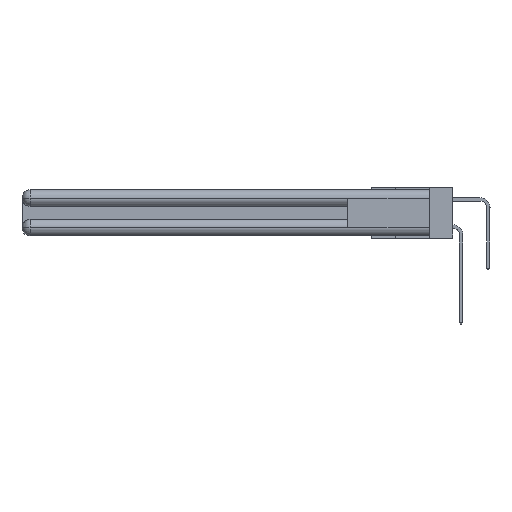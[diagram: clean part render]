
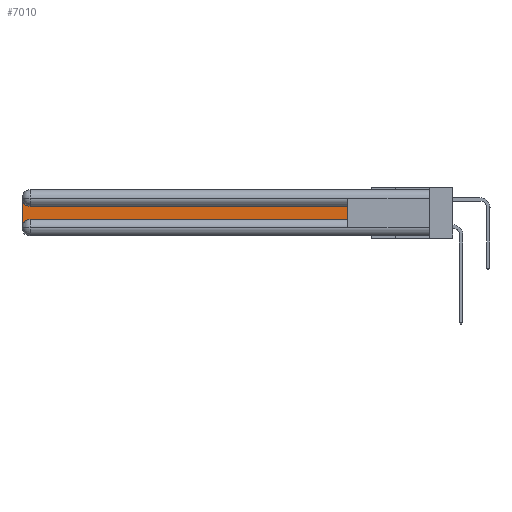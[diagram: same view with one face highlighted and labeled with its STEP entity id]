
A CAD part, left-side view. The second image highlights one B-rep face of the part: STEP entity #7010.
In plain terms, the highlighted planar face has unit normal (-1, 0, 0).
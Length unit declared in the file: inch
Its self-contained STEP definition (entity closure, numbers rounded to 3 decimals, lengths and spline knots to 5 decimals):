
#18 = DIRECTION ( 'NONE',  ( 1., 0., 0. ) ) ;
#355 = CARTESIAN_POINT ( 'NONE',  ( 0.075, 2.94, -0.2775 ) ) ;
#578 = CARTESIAN_POINT ( 'NONE',  ( 0.075, 2.94, -0.2175 ) ) ;
#766 = ORIENTED_EDGE ( 'NONE', *, *, #27899, .T. ) ;
#861 = EDGE_CURVE ( 'NONE', #5225, #5058, #1447, .T. ) ;
#911 = EDGE_CURVE ( 'NONE', #29922, #8010, #19215, .T. ) ;
#1120 = EDGE_CURVE ( 'NONE', #6606, #12666, #27124, .T. ) ;
#1179 = DIRECTION ( 'NONE',  ( 0., 0., 1. ) ) ;
#1447 = CIRCLE ( 'NONE', #16295, 0.06 ) ;
#1865 = CARTESIAN_POINT ( 'NONE',  ( 0.075, 3., -0.2175 ) ) ;
#2793 = DIRECTION ( 'NONE',  ( 1., 0., 0. ) ) ;
#4645 = ORIENTED_EDGE ( 'NONE', *, *, #19676, .T. ) ;
#4651 = FACE_OUTER_BOUND ( 'NONE', #5814, .T. ) ;
#5058 = VERTEX_POINT ( 'NONE', #7062 ) ;
#5225 = VERTEX_POINT ( 'NONE', #29302 ) ;
#5548 = DIRECTION ( 'NONE',  ( 0., 1., 0. ) ) ;
#5814 = EDGE_LOOP ( 'NONE', ( #4645, #27393, #766, #28518, #8249, #23352 ) ) ;
#6006 = CARTESIAN_POINT ( 'NONE',  ( 0.075, 0.6, -0.2175 ) ) ;
#6606 = VERTEX_POINT ( 'NONE', #13624 ) ;
#7010 = ADVANCED_FACE ( 'NONE', ( #4651 ), #20815, .F. ) ;
#7062 = CARTESIAN_POINT ( 'NONE',  ( 0.075, 3., -0.0625 ) ) ;
#8010 = VERTEX_POINT ( 'NONE', #578 ) ;
#8151 = AXIS2_PLACEMENT_3D ( 'NONE', #23577, #18272, #28086 ) ;
#8249 = ORIENTED_EDGE ( 'NONE', *, *, #24310, .T. ) ;
#9406 = CARTESIAN_POINT ( 'NONE',  ( 0.075, 3., -0.2775 ) ) ;
#11035 = VECTOR ( 'NONE', #5548, 39.37008 ) ;
#12666 = VERTEX_POINT ( 'NONE', #16071 ) ;
#13624 = CARTESIAN_POINT ( 'NONE',  ( 0.075, 0.6, -0.2175 ) ) ;
#16071 = CARTESIAN_POINT ( 'NONE',  ( 0.075, 0.6, -0.1225 ) ) ;
#16295 = AXIS2_PLACEMENT_3D ( 'NONE', #29096, #18, #22030 ) ;
#18272 = DIRECTION ( 'NONE',  ( 1., 0., 0. ) ) ;
#19215 = CIRCLE ( 'NONE', #22332, 0.06 ) ;
#19676 = EDGE_CURVE ( 'NONE', #12666, #5225, #26894, .T. ) ;
#20035 = CARTESIAN_POINT ( 'NONE',  ( 0.075, 0.6, -0.1225 ) ) ;
#20189 = LINE ( 'NONE', #24425, #22486 ) ;
#20815 = PLANE ( 'NONE',  #8151 ) ;
#21258 = LINE ( 'NONE', #1865, #27285 ) ;
#21796 = DIRECTION ( 'NONE',  ( 0., -1., 0. ) ) ;
#22030 = DIRECTION ( 'NONE',  ( 0., 0., -1. ) ) ;
#22134 = DIRECTION ( 'NONE',  ( 0., 0., -1. ) ) ;
#22332 = AXIS2_PLACEMENT_3D ( 'NONE', #355, #2793, #22134 ) ;
#22486 = VECTOR ( 'NONE', #21796, 39.37008 ) ;
#23352 = ORIENTED_EDGE ( 'NONE', *, *, #1120, .T. ) ;
#23577 = CARTESIAN_POINT ( 'NONE',  ( 0.075, 3., -0.1225 ) ) ;
#24098 = VECTOR ( 'NONE', #1179, 39.37008 ) ;
#24310 = EDGE_CURVE ( 'NONE', #8010, #6606, #20189, .T. ) ;
#24425 = CARTESIAN_POINT ( 'NONE',  ( 0.075, 0.6, -0.2175 ) ) ;
#26459 = DIRECTION ( 'NONE',  ( 0., 0., -1. ) ) ;
#26894 = LINE ( 'NONE', #20035, #11035 ) ;
#27124 = LINE ( 'NONE', #6006, #24098 ) ;
#27285 = VECTOR ( 'NONE', #26459, 39.37008 ) ;
#27393 = ORIENTED_EDGE ( 'NONE', *, *, #861, .T. ) ;
#27899 = EDGE_CURVE ( 'NONE', #5058, #29922, #21258, .T. ) ;
#28086 = DIRECTION ( 'NONE',  ( 0., 0., -1. ) ) ;
#28518 = ORIENTED_EDGE ( 'NONE', *, *, #911, .T. ) ;
#29096 = CARTESIAN_POINT ( 'NONE',  ( 0.075, 2.94, -0.0625 ) ) ;
#29302 = CARTESIAN_POINT ( 'NONE',  ( 0.075, 2.94, -0.1225 ) ) ;
#29922 = VERTEX_POINT ( 'NONE', #9406 ) ;
